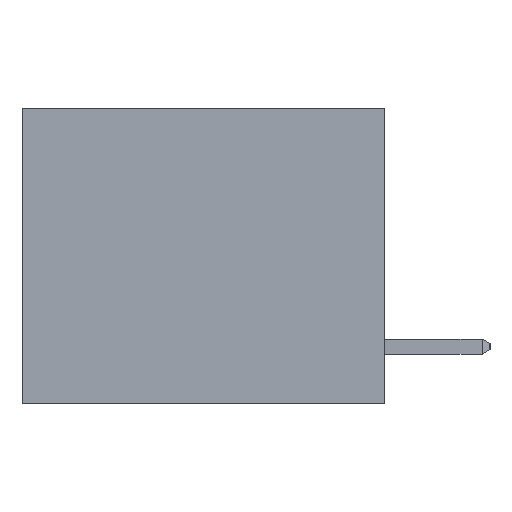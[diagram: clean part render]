
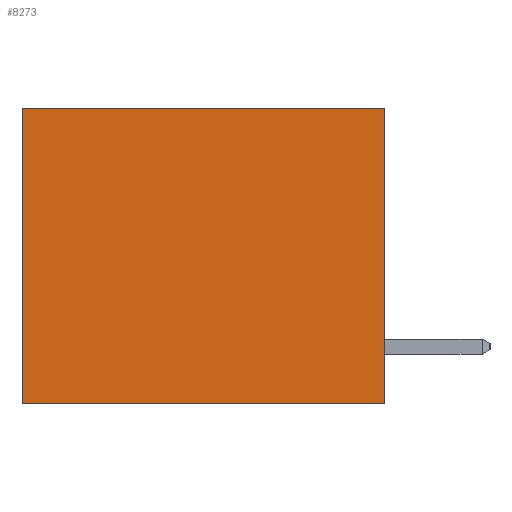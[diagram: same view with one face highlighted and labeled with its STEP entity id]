
A CAD part, left-side view. The second image highlights one B-rep face of the part: STEP entity #8273.
In plain terms, the highlighted planar face has unit normal (-1, 0, 0).
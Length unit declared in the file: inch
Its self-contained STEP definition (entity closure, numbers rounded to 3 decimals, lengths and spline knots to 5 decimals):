
#1039 = LINE ( 'NONE', #12645, #4274 ) ;
#1894 = EDGE_CURVE ( 'NONE', #3727, #5416, #11316, .T. ) ;
#2047 = DIRECTION ( 'NONE',  ( 0., 0., -1. ) ) ;
#2551 = FACE_OUTER_BOUND ( 'NONE', #12019, .T. ) ;
#3727 = VERTEX_POINT ( 'NONE', #19667 ) ;
#4274 = VECTOR ( 'NONE', #2047, 39.37008 ) ;
#4435 = EDGE_CURVE ( 'NONE', #14662, #20639, #4988, .T. ) ;
#4940 = ORIENTED_EDGE ( 'NONE', *, *, #14571, .F. ) ;
#4988 = LINE ( 'NONE', #17532, #14462 ) ;
#5416 = VERTEX_POINT ( 'NONE', #7044 ) ;
#6610 = CARTESIAN_POINT ( 'NONE',  ( 0.3165, 0., 0. ) ) ;
#7044 = CARTESIAN_POINT ( 'NONE',  ( 0.3165, 0.6, -0.49 ) ) ;
#8273 = ADVANCED_FACE ( 'NONE', ( #2551 ), #21174, .F. ) ;
#8372 = ORIENTED_EDGE ( 'NONE', *, *, #4435, .T. ) ;
#8692 = DIRECTION ( 'NONE',  ( 0., 0., -1. ) ) ;
#10861 = CARTESIAN_POINT ( 'NONE',  ( 0.3165, 0., -0.49 ) ) ;
#11316 = LINE ( 'NONE', #13745, #11979 ) ;
#11979 = VECTOR ( 'NONE', #13654, 39.37008 ) ;
#12019 = EDGE_LOOP ( 'NONE', ( #23035, #19018, #4940, #8372 ) ) ;
#12645 = CARTESIAN_POINT ( 'NONE',  ( 0.3165, 0., -0.49 ) ) ;
#12879 = DIRECTION ( 'NONE',  ( 0., 0., -1. ) ) ;
#13238 = EDGE_CURVE ( 'NONE', #20639, #5416, #16420, .T. ) ;
#13654 = DIRECTION ( 'NONE',  ( 0., 1., 0. ) ) ;
#13745 = CARTESIAN_POINT ( 'NONE',  ( 0.3165, 0., -0.49 ) ) ;
#14462 = VECTOR ( 'NONE', #19450, 39.37008 ) ;
#14571 = EDGE_CURVE ( 'NONE', #14662, #3727, #1039, .T. ) ;
#14662 = VERTEX_POINT ( 'NONE', #6610 ) ;
#16420 = LINE ( 'NONE', #23519, #21613 ) ;
#17532 = CARTESIAN_POINT ( 'NONE',  ( 0.3165, 0., 0. ) ) ;
#19018 = ORIENTED_EDGE ( 'NONE', *, *, #1894, .F. ) ;
#19085 = DIRECTION ( 'NONE',  ( 1., 0., 0. ) ) ;
#19261 = CARTESIAN_POINT ( 'NONE',  ( 0.3165, 0.6, 0. ) ) ;
#19450 = DIRECTION ( 'NONE',  ( 0., 1., 0. ) ) ;
#19667 = CARTESIAN_POINT ( 'NONE',  ( 0.3165, 0., -0.49 ) ) ;
#20639 = VERTEX_POINT ( 'NONE', #19261 ) ;
#21174 = PLANE ( 'NONE',  #22156 ) ;
#21613 = VECTOR ( 'NONE', #12879, 39.37008 ) ;
#22156 = AXIS2_PLACEMENT_3D ( 'NONE', #10861, #19085, #8692 ) ;
#23035 = ORIENTED_EDGE ( 'NONE', *, *, #13238, .T. ) ;
#23519 = CARTESIAN_POINT ( 'NONE',  ( 0.3165, 0.6, -0.49 ) ) ;
